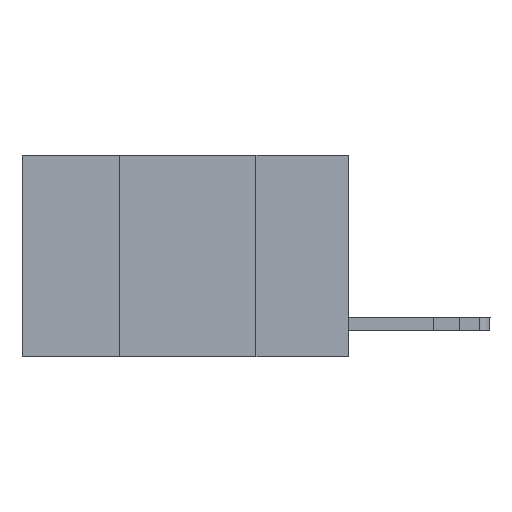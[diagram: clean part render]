
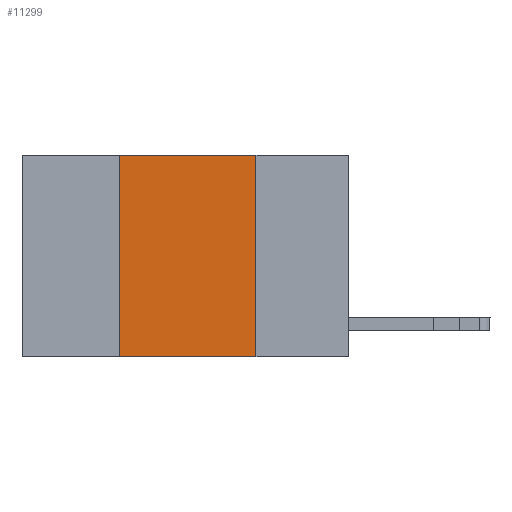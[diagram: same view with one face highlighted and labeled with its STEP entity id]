
A CAD part, left-side view. The second image highlights one B-rep face of the part: STEP entity #11299.
In plain terms, the highlighted planar face has unit normal (-1, 0, 0).
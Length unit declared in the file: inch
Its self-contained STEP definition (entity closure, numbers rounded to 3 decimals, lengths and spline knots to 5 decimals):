
#1742 = EDGE_CURVE ( 'NONE', #5872, #11834, #7752, .T. ) ;
#3353 = ORIENTED_EDGE ( 'NONE', *, *, #4365, .F. ) ;
#3432 = DIRECTION ( 'NONE',  ( 0., 0., -1. ) ) ;
#3905 = VECTOR ( 'NONE', #18824, 39.37008 ) ;
#4365 = EDGE_CURVE ( 'NONE', #5872, #6947, #10130, .T. ) ;
#5536 = CARTESIAN_POINT ( 'NONE',  ( 0., 0.42, 0. ) ) ;
#5603 = VECTOR ( 'NONE', #18252, 39.37008 ) ;
#5872 = VERTEX_POINT ( 'NONE', #6284 ) ;
#6284 = CARTESIAN_POINT ( 'NONE',  ( 0., 0.42, -0.37 ) ) ;
#6297 = CARTESIAN_POINT ( 'NONE',  ( 0., 0.17, -0.37 ) ) ;
#6854 = CARTESIAN_POINT ( 'NONE',  ( 0., 0.17, 0. ) ) ;
#6947 = VERTEX_POINT ( 'NONE', #19868 ) ;
#7620 = VERTEX_POINT ( 'NONE', #16360 ) ;
#7752 = LINE ( 'NONE', #8017, #7794 ) ;
#7794 = VECTOR ( 'NONE', #26144, 39.37008 ) ;
#8017 = CARTESIAN_POINT ( 'NONE',  ( 0., 0.6, -0.37 ) ) ;
#8525 = EDGE_CURVE ( 'NONE', #7620, #11834, #8844, .T. ) ;
#8844 = LINE ( 'NONE', #6854, #3905 ) ;
#10130 = LINE ( 'NONE', #5536, #5603 ) ;
#10522 = EDGE_LOOP ( 'NONE', ( #25043, #11813, #3353, #23384 ) ) ;
#10851 = CARTESIAN_POINT ( 'NONE',  ( 0., 0.6, 0. ) ) ;
#11299 = ADVANCED_FACE ( 'NONE', ( #23557 ), #21554, .F. ) ;
#11813 = ORIENTED_EDGE ( 'NONE', *, *, #16047, .F. ) ;
#11834 = VERTEX_POINT ( 'NONE', #6297 ) ;
#16047 = EDGE_CURVE ( 'NONE', #6947, #7620, #23122, .T. ) ;
#16360 = CARTESIAN_POINT ( 'NONE',  ( 0., 0.17, 0. ) ) ;
#18252 = DIRECTION ( 'NONE',  ( 0., 0., 1. ) ) ;
#18824 = DIRECTION ( 'NONE',  ( 0., 0., -1. ) ) ;
#18982 = DIRECTION ( 'NONE',  ( 0., -1., 0. ) ) ;
#19868 = CARTESIAN_POINT ( 'NONE',  ( 0., 0.42, 0. ) ) ;
#21034 = AXIS2_PLACEMENT_3D ( 'NONE', #25700, #25829, #3432 ) ;
#21554 = PLANE ( 'NONE',  #21034 ) ;
#21567 = VECTOR ( 'NONE', #18982, 39.37008 ) ;
#23122 = LINE ( 'NONE', #10851, #21567 ) ;
#23384 = ORIENTED_EDGE ( 'NONE', *, *, #1742, .T. ) ;
#23557 = FACE_OUTER_BOUND ( 'NONE', #10522, .T. ) ;
#25043 = ORIENTED_EDGE ( 'NONE', *, *, #8525, .F. ) ;
#25700 = CARTESIAN_POINT ( 'NONE',  ( 0., 0.6, 0. ) ) ;
#25829 = DIRECTION ( 'NONE',  ( 1., 0., 0. ) ) ;
#26144 = DIRECTION ( 'NONE',  ( 0., -1., 0. ) ) ;
